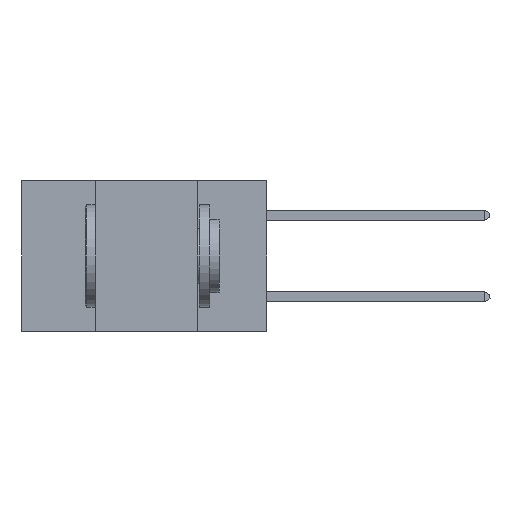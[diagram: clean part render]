
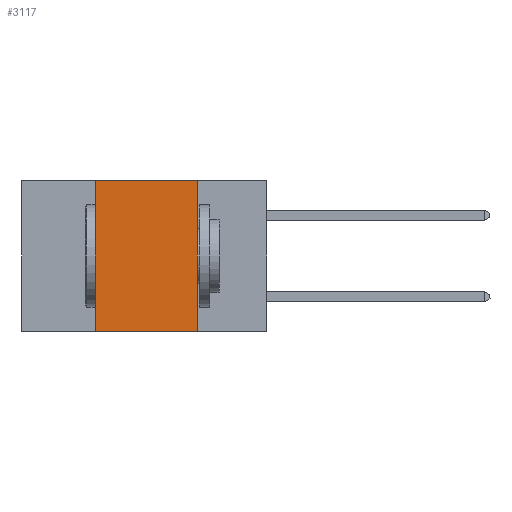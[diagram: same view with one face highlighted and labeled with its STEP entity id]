
A CAD part, left-side view. The second image highlights one B-rep face of the part: STEP entity #3117.
In plain terms, the highlighted planar face has unit normal (-1, 0, 0).
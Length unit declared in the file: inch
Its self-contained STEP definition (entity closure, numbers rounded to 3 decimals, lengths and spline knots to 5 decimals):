
#13 = DIRECTION ( 'NONE',  ( 0., 0., 1. ) ) ;
#1491 = DIRECTION ( 'NONE',  ( 0., 0., -1. ) ) ;
#1500 = DIRECTION ( 'NONE',  ( 1., 0., 0. ) ) ;
#1539 = DIRECTION ( 'NONE',  ( 0., 0., -1. ) ) ;
#1554 = CARTESIAN_POINT ( 'NONE',  ( 0., 0.6, 0. ) ) ;
#1576 = PLANE ( 'NONE',  #7206 ) ;
#1747 = DIRECTION ( 'NONE',  ( 0., -1., 0. ) ) ;
#1906 = VECTOR ( 'NONE', #2682, 39.37008 ) ;
#2331 = ORIENTED_EDGE ( 'NONE', *, *, #22272, .F. ) ;
#2682 = DIRECTION ( 'NONE',  ( 0., -1., 0. ) ) ;
#2971 = CARTESIAN_POINT ( 'NONE',  ( 0., 0.42, 0. ) ) ;
#3117 = ADVANCED_FACE ( 'NONE', ( #7723 ), #1576, .F. ) ;
#3400 = EDGE_CURVE ( 'NONE', #13715, #13102, #11059, .T. ) ;
#4965 = ORIENTED_EDGE ( 'NONE', *, *, #9562, .F. ) ;
#5389 = ORIENTED_EDGE ( 'NONE', *, *, #3400, .F. ) ;
#5570 = CARTESIAN_POINT ( 'NONE',  ( 0., 0.42, 0. ) ) ;
#7031 = LINE ( 'NONE', #7264, #20097 ) ;
#7206 = AXIS2_PLACEMENT_3D ( 'NONE', #1554, #1500, #1491 ) ;
#7264 = CARTESIAN_POINT ( 'NONE',  ( 0., 0.6, -0.37 ) ) ;
#7663 = VECTOR ( 'NONE', #1539, 39.37008 ) ;
#7723 = FACE_OUTER_BOUND ( 'NONE', #19336, .T. ) ;
#9562 = EDGE_CURVE ( 'NONE', #13102, #18748, #17644, .T. ) ;
#10665 = CARTESIAN_POINT ( 'NONE',  ( 0., 0.17, 0. ) ) ;
#11059 = LINE ( 'NONE', #11775, #1906 ) ;
#11775 = CARTESIAN_POINT ( 'NONE',  ( 0., 0.6, 0. ) ) ;
#13073 = VERTEX_POINT ( 'NONE', #19123 ) ;
#13102 = VERTEX_POINT ( 'NONE', #17331 ) ;
#13715 = VERTEX_POINT ( 'NONE', #2971 ) ;
#14387 = LINE ( 'NONE', #5570, #17975 ) ;
#15622 = CARTESIAN_POINT ( 'NONE',  ( 0., 0.17, -0.37 ) ) ;
#16979 = EDGE_CURVE ( 'NONE', #13073, #18748, #7031, .T. ) ;
#17331 = CARTESIAN_POINT ( 'NONE',  ( 0., 0.17, 0. ) ) ;
#17644 = LINE ( 'NONE', #10665, #7663 ) ;
#17975 = VECTOR ( 'NONE', #13, 39.37008 ) ;
#18748 = VERTEX_POINT ( 'NONE', #15622 ) ;
#19123 = CARTESIAN_POINT ( 'NONE',  ( 0., 0.42, -0.37 ) ) ;
#19336 = EDGE_LOOP ( 'NONE', ( #4965, #5389, #2331, #20073 ) ) ;
#20073 = ORIENTED_EDGE ( 'NONE', *, *, #16979, .T. ) ;
#20097 = VECTOR ( 'NONE', #1747, 39.37008 ) ;
#22272 = EDGE_CURVE ( 'NONE', #13073, #13715, #14387, .T. ) ;
